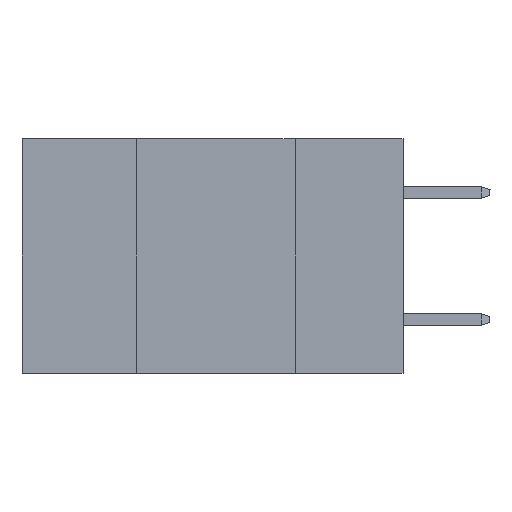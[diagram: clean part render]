
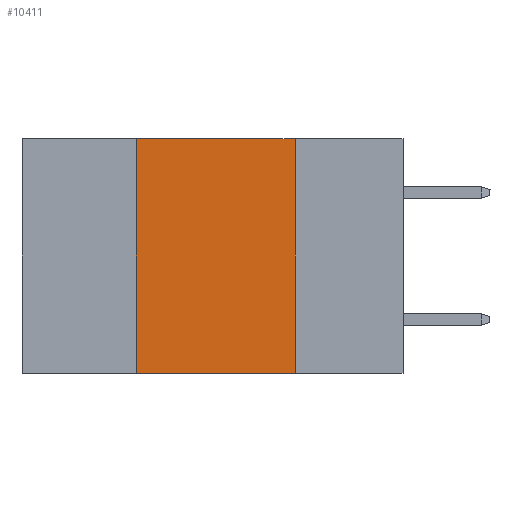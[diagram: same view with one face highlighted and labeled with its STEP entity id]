
A CAD part, left-side view. The second image highlights one B-rep face of the part: STEP entity #10411.
In plain terms, the highlighted planar face has unit normal (-1, 0, 0).
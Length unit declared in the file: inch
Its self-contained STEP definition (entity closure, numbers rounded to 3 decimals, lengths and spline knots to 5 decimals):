
#485 = ORIENTED_EDGE ( 'NONE', *, *, #7133, .T. ) ;
#817 = ORIENTED_EDGE ( 'NONE', *, *, #16134, .F. ) ;
#1109 = EDGE_CURVE ( 'NONE', #19897, #17531, #19613, .T. ) ;
#1993 = CARTESIAN_POINT ( 'NONE',  ( 0., 0.6, 0. ) ) ;
#2113 = DIRECTION ( 'NONE',  ( 0., 0., -1. ) ) ;
#2589 = VECTOR ( 'NONE', #5426, 39.37008 ) ;
#5426 = DIRECTION ( 'NONE',  ( 0., -1., 0. ) ) ;
#6674 = CARTESIAN_POINT ( 'NONE',  ( 0., 0.6, -0.37 ) ) ;
#6681 = LINE ( 'NONE', #8236, #18504 ) ;
#6697 = VERTEX_POINT ( 'NONE', #12583 ) ;
#7133 = EDGE_CURVE ( 'NONE', #19897, #6697, #9785, .T. ) ;
#8172 = CARTESIAN_POINT ( 'NONE',  ( 0., 0.17, 0. ) ) ;
#8224 = DIRECTION ( 'NONE',  ( 1., 0., 0. ) ) ;
#8236 = CARTESIAN_POINT ( 'NONE',  ( 0., 0.17, 0. ) ) ;
#8325 = DIRECTION ( 'NONE',  ( 0., 0., -1. ) ) ;
#9677 = PLANE ( 'NONE',  #11608 ) ;
#9785 = LINE ( 'NONE', #6674, #16074 ) ;
#10165 = LINE ( 'NONE', #19447, #2589 ) ;
#10411 = ADVANCED_FACE ( 'NONE', ( #16065 ), #9677, .F. ) ;
#11198 = EDGE_LOOP ( 'NONE', ( #817, #11983, #18505, #485 ) ) ;
#11491 = DIRECTION ( 'NONE',  ( 0., -1., 0. ) ) ;
#11608 = AXIS2_PLACEMENT_3D ( 'NONE', #1993, #8224, #8325 ) ;
#11983 = ORIENTED_EDGE ( 'NONE', *, *, #15630, .F. ) ;
#12583 = CARTESIAN_POINT ( 'NONE',  ( 0., 0.17, -0.37 ) ) ;
#13583 = CARTESIAN_POINT ( 'NONE',  ( 0., 0.42, 0. ) ) ;
#14194 = CARTESIAN_POINT ( 'NONE',  ( 0., 0.42, -0.37 ) ) ;
#15630 = EDGE_CURVE ( 'NONE', #17531, #18291, #10165, .T. ) ;
#16065 = FACE_OUTER_BOUND ( 'NONE', #11198, .T. ) ;
#16074 = VECTOR ( 'NONE', #11491, 39.37008 ) ;
#16134 = EDGE_CURVE ( 'NONE', #18291, #6697, #6681, .T. ) ;
#16325 = DIRECTION ( 'NONE',  ( 0., 0., 1. ) ) ;
#17531 = VERTEX_POINT ( 'NONE', #13583 ) ;
#18248 = VECTOR ( 'NONE', #16325, 39.37008 ) ;
#18291 = VERTEX_POINT ( 'NONE', #8172 ) ;
#18504 = VECTOR ( 'NONE', #2113, 39.37008 ) ;
#18505 = ORIENTED_EDGE ( 'NONE', *, *, #1109, .F. ) ;
#19447 = CARTESIAN_POINT ( 'NONE',  ( 0., 0.6, 0. ) ) ;
#19516 = CARTESIAN_POINT ( 'NONE',  ( 0., 0.42, 0. ) ) ;
#19613 = LINE ( 'NONE', #19516, #18248 ) ;
#19897 = VERTEX_POINT ( 'NONE', #14194 ) ;
